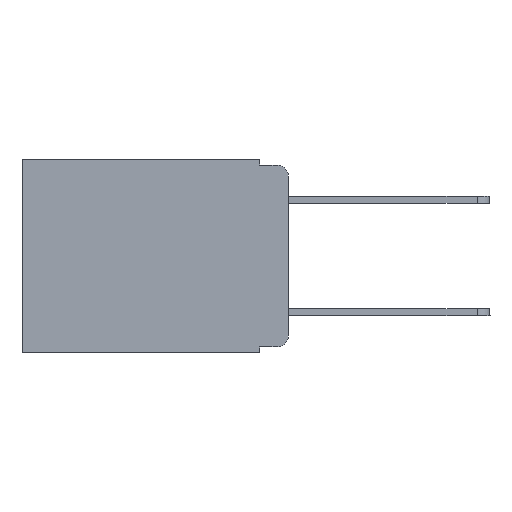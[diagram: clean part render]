
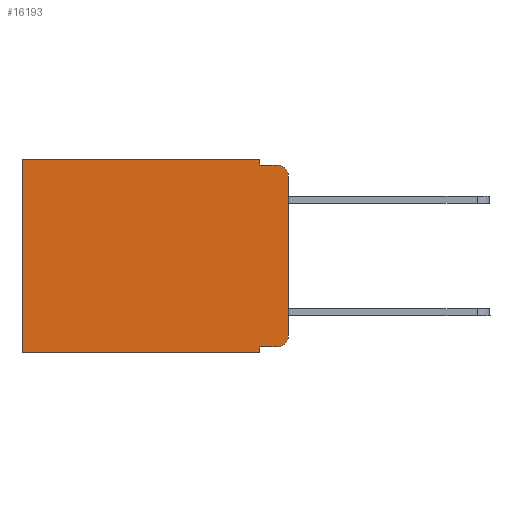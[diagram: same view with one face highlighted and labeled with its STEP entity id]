
A CAD part, left-side view. The second image highlights one B-rep face of the part: STEP entity #16193.
In plain terms, the highlighted planar face has unit normal (-1, 0, 0).
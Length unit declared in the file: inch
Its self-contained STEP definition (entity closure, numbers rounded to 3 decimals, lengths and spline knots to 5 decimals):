
#961 = CARTESIAN_POINT ( 'NONE',  ( 0.298, 0.02, -0.333 ) ) ;
#1068 = EDGE_CURVE ( 'NONE', #12872, #23902, #16499, .T. ) ;
#1493 = VECTOR ( 'NONE', #12250, 39.37008 ) ;
#1495 = EDGE_CURVE ( 'NONE', #18523, #1872, #9835, .T. ) ;
#1501 = VECTOR ( 'NONE', #13778, 39.37008 ) ;
#1872 = VERTEX_POINT ( 'NONE', #17610 ) ;
#2399 = CARTESIAN_POINT ( 'NONE',  ( 0.298, 0.051, 0. ) ) ;
#2412 = CARTESIAN_POINT ( 'NONE',  ( 0.298, 0., 0. ) ) ;
#2465 = CARTESIAN_POINT ( 'NONE',  ( 0.298, 0., -0.03 ) ) ;
#2729 = DIRECTION ( 'NONE',  ( 0., 0., -1. ) ) ;
#2731 = CARTESIAN_POINT ( 'NONE',  ( 0.298, 0.02, -0.01 ) ) ;
#3055 = EDGE_LOOP ( 'NONE', ( #3533, #17779, #12149, #11572, #20001, #23247, #4128, #21134, #22264, #19690 ) ) ;
#3533 = ORIENTED_EDGE ( 'NONE', *, *, #10943, .F. ) ;
#4104 = DIRECTION ( 'NONE',  ( 0., -1., 0. ) ) ;
#4128 = ORIENTED_EDGE ( 'NONE', *, *, #21945, .F. ) ;
#4178 = VERTEX_POINT ( 'NONE', #2465 ) ;
#4181 = LINE ( 'NONE', #16287, #16082 ) ;
#4214 = CARTESIAN_POINT ( 'NONE',  ( 0.298, 0., -0.343 ) ) ;
#4458 = LINE ( 'NONE', #4214, #15510 ) ;
#5279 = EDGE_CURVE ( 'NONE', #20113, #12872, #18403, .T. ) ;
#5315 = VERTEX_POINT ( 'NONE', #12351 ) ;
#5493 = CARTESIAN_POINT ( 'NONE',  ( 0.298, 0.02, -0.313 ) ) ;
#5660 = DIRECTION ( 'NONE',  ( 1., 0., 0. ) ) ;
#6026 = CARTESIAN_POINT ( 'NONE',  ( 0.298, 0., 0. ) ) ;
#6426 = LINE ( 'NONE', #17378, #1493 ) ;
#6841 = EDGE_CURVE ( 'NONE', #20113, #23116, #8766, .T. ) ;
#7468 = CARTESIAN_POINT ( 'NONE',  ( 0.298, 0.473, -0.343 ) ) ;
#7968 = EDGE_CURVE ( 'NONE', #9915, #18523, #12564, .T. ) ;
#8245 = CARTESIAN_POINT ( 'NONE',  ( 0.298, 0.051, -0.01 ) ) ;
#8766 = LINE ( 'NONE', #6026, #1501 ) ;
#8966 = AXIS2_PLACEMENT_3D ( 'NONE', #22268, #5660, #18610 ) ;
#9213 = PLANE ( 'NONE',  #8966 ) ;
#9835 = CIRCLE ( 'NONE', #10673, 0.02 ) ;
#9915 = VERTEX_POINT ( 'NONE', #23431 ) ;
#10275 = FACE_OUTER_BOUND ( 'NONE', #3055, .T. ) ;
#10673 = AXIS2_PLACEMENT_3D ( 'NONE', #5493, #22118, #22273 ) ;
#10943 = EDGE_CURVE ( 'NONE', #4178, #1872, #17130, .T. ) ;
#11544 = EDGE_CURVE ( 'NONE', #9915, #5315, #6426, .T. ) ;
#11572 = ORIENTED_EDGE ( 'NONE', *, *, #5279, .F. ) ;
#12149 = ORIENTED_EDGE ( 'NONE', *, *, #1068, .F. ) ;
#12250 = DIRECTION ( 'NONE',  ( 0., 0., -1. ) ) ;
#12351 = CARTESIAN_POINT ( 'NONE',  ( 0.298, 0.051, -0.343 ) ) ;
#12564 = LINE ( 'NONE', #19540, #13202 ) ;
#12696 = VERTEX_POINT ( 'NONE', #7468 ) ;
#12742 = AXIS2_PLACEMENT_3D ( 'NONE', #18022, #20066, #17859 ) ;
#12872 = VERTEX_POINT ( 'NONE', #8245 ) ;
#13202 = VECTOR ( 'NONE', #17736, 39.37008 ) ;
#13626 = DIRECTION ( 'NONE',  ( 0., 0., -1. ) ) ;
#13778 = DIRECTION ( 'NONE',  ( 0., 1., 0. ) ) ;
#13810 = CARTESIAN_POINT ( 'NONE',  ( 0.298, 0.051, 0. ) ) ;
#13833 = CARTESIAN_POINT ( 'NONE',  ( 0.298, 0.473, 0. ) ) ;
#14474 = VECTOR ( 'NONE', #4104, 39.37008 ) ;
#15510 = VECTOR ( 'NONE', #19276, 39.37008 ) ;
#16058 = EDGE_CURVE ( 'NONE', #23116, #12696, #4181, .T. ) ;
#16082 = VECTOR ( 'NONE', #18045, 39.37008 ) ;
#16193 = ADVANCED_FACE ( 'NONE', ( #10275 ), #9213, .F. ) ;
#16287 = CARTESIAN_POINT ( 'NONE',  ( 0.298, 0.473, 0. ) ) ;
#16349 = CARTESIAN_POINT ( 'NONE',  ( 0.298, 0.051, -0.01 ) ) ;
#16499 = LINE ( 'NONE', #16349, #14474 ) ;
#16953 = CIRCLE ( 'NONE', #12742, 0.02 ) ;
#17130 = LINE ( 'NONE', #2412, #19468 ) ;
#17378 = CARTESIAN_POINT ( 'NONE',  ( 0.298, 0.051, 0. ) ) ;
#17610 = CARTESIAN_POINT ( 'NONE',  ( 0.298, 0., -0.313 ) ) ;
#17736 = DIRECTION ( 'NONE',  ( 0., -1., 0. ) ) ;
#17779 = ORIENTED_EDGE ( 'NONE', *, *, #21624, .T. ) ;
#17859 = DIRECTION ( 'NONE',  ( 0., 0., -1. ) ) ;
#18022 = CARTESIAN_POINT ( 'NONE',  ( 0.298, 0.02, -0.03 ) ) ;
#18045 = DIRECTION ( 'NONE',  ( 0., 0., -1. ) ) ;
#18403 = LINE ( 'NONE', #13810, #23930 ) ;
#18523 = VERTEX_POINT ( 'NONE', #961 ) ;
#18610 = DIRECTION ( 'NONE',  ( 0., 0., -1. ) ) ;
#19276 = DIRECTION ( 'NONE',  ( 0., 1., 0. ) ) ;
#19468 = VECTOR ( 'NONE', #13626, 39.37008 ) ;
#19540 = CARTESIAN_POINT ( 'NONE',  ( 0.298, 0.051, -0.333 ) ) ;
#19690 = ORIENTED_EDGE ( 'NONE', *, *, #1495, .T. ) ;
#20001 = ORIENTED_EDGE ( 'NONE', *, *, #6841, .T. ) ;
#20066 = DIRECTION ( 'NONE',  ( -1., 0., 0. ) ) ;
#20113 = VERTEX_POINT ( 'NONE', #2399 ) ;
#21134 = ORIENTED_EDGE ( 'NONE', *, *, #11544, .F. ) ;
#21624 = EDGE_CURVE ( 'NONE', #4178, #23902, #16953, .T. ) ;
#21945 = EDGE_CURVE ( 'NONE', #5315, #12696, #4458, .T. ) ;
#22118 = DIRECTION ( 'NONE',  ( -1., 0., 0. ) ) ;
#22264 = ORIENTED_EDGE ( 'NONE', *, *, #7968, .T. ) ;
#22268 = CARTESIAN_POINT ( 'NONE',  ( 0.298, 0., 0. ) ) ;
#22273 = DIRECTION ( 'NONE',  ( 0., 0., -1. ) ) ;
#23116 = VERTEX_POINT ( 'NONE', #13833 ) ;
#23247 = ORIENTED_EDGE ( 'NONE', *, *, #16058, .T. ) ;
#23431 = CARTESIAN_POINT ( 'NONE',  ( 0.298, 0.051, -0.333 ) ) ;
#23902 = VERTEX_POINT ( 'NONE', #2731 ) ;
#23930 = VECTOR ( 'NONE', #2729, 39.37008 ) ;
